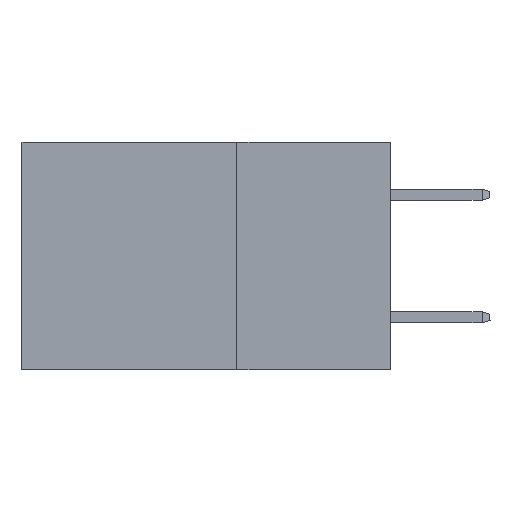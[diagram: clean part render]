
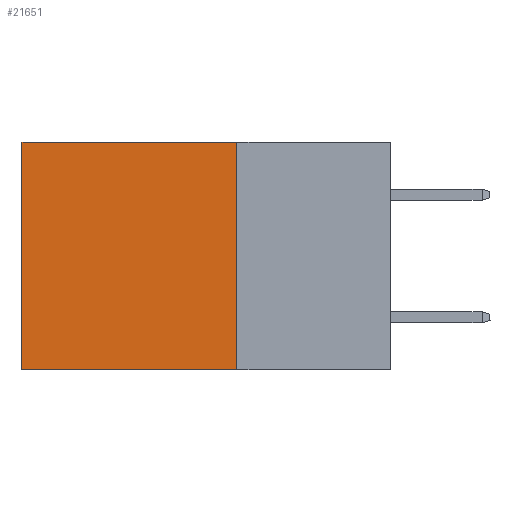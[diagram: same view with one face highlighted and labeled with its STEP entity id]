
A CAD part, left-side view. The second image highlights one B-rep face of the part: STEP entity #21651.
In plain terms, the highlighted planar face has unit normal (-1, 0, 0).
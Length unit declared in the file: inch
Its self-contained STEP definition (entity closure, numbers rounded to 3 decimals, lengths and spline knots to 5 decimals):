
#86 = AXIS2_PLACEMENT_3D ( 'NONE', #5523, #19975, #308 ) ;
#308 = DIRECTION ( 'NONE',  ( 0., 0., -1. ) ) ;
#914 = VECTOR ( 'NONE', #21416, 39.37008 ) ;
#2972 = LINE ( 'NONE', #5788, #22407 ) ;
#4132 = VERTEX_POINT ( 'NONE', #22344 ) ;
#5523 = CARTESIAN_POINT ( 'NONE',  ( 0.2875, 0.25, 0. ) ) ;
#5662 = VERTEX_POINT ( 'NONE', #13096 ) ;
#5788 = CARTESIAN_POINT ( 'NONE',  ( 0.2875, 0.25, 0. ) ) ;
#7143 = ORIENTED_EDGE ( 'NONE', *, *, #9654, .T. ) ;
#7528 = VECTOR ( 'NONE', #22799, 39.37008 ) ;
#8505 = FACE_OUTER_BOUND ( 'NONE', #16741, .T. ) ;
#9654 = EDGE_CURVE ( 'NONE', #4132, #20805, #18664, .T. ) ;
#10440 = LINE ( 'NONE', #16148, #914 ) ;
#11609 = VECTOR ( 'NONE', #16174, 39.37008 ) ;
#12291 = LINE ( 'NONE', #21137, #7528 ) ;
#13096 = CARTESIAN_POINT ( 'NONE',  ( 0.2875, 0.25, 0. ) ) ;
#13514 = CARTESIAN_POINT ( 'NONE',  ( 0.2875, 0.25, -0.37 ) ) ;
#13671 = EDGE_CURVE ( 'NONE', #20940, #20805, #12291, .T. ) ;
#13829 = ORIENTED_EDGE ( 'NONE', *, *, #21340, .T. ) ;
#16148 = CARTESIAN_POINT ( 'NONE',  ( 0.2875, 0.25, 0. ) ) ;
#16174 = DIRECTION ( 'NONE',  ( 0., 0., -1. ) ) ;
#16357 = PLANE ( 'NONE',  #86 ) ;
#16741 = EDGE_LOOP ( 'NONE', ( #7143, #21560, #21030, #13829 ) ) ;
#17116 = EDGE_CURVE ( 'NONE', #5662, #20940, #2972, .T. ) ;
#18198 = CARTESIAN_POINT ( 'NONE',  ( 0.2875, 0.6, -0.37 ) ) ;
#18277 = CARTESIAN_POINT ( 'NONE',  ( 0.2875, 0.6, 0. ) ) ;
#18664 = LINE ( 'NONE', #18277, #11609 ) ;
#19975 = DIRECTION ( 'NONE',  ( 1., 0., 0. ) ) ;
#20203 = DIRECTION ( 'NONE',  ( 0., 0., -1. ) ) ;
#20805 = VERTEX_POINT ( 'NONE', #18198 ) ;
#20940 = VERTEX_POINT ( 'NONE', #13514 ) ;
#21030 = ORIENTED_EDGE ( 'NONE', *, *, #17116, .F. ) ;
#21137 = CARTESIAN_POINT ( 'NONE',  ( 0.2875, 0.25, -0.37 ) ) ;
#21340 = EDGE_CURVE ( 'NONE', #5662, #4132, #10440, .T. ) ;
#21416 = DIRECTION ( 'NONE',  ( 0., 1., 0. ) ) ;
#21560 = ORIENTED_EDGE ( 'NONE', *, *, #13671, .F. ) ;
#21651 = ADVANCED_FACE ( 'NONE', ( #8505 ), #16357, .F. ) ;
#22344 = CARTESIAN_POINT ( 'NONE',  ( 0.2875, 0.6, 0. ) ) ;
#22407 = VECTOR ( 'NONE', #20203, 39.37008 ) ;
#22799 = DIRECTION ( 'NONE',  ( 0., 1., 0. ) ) ;
